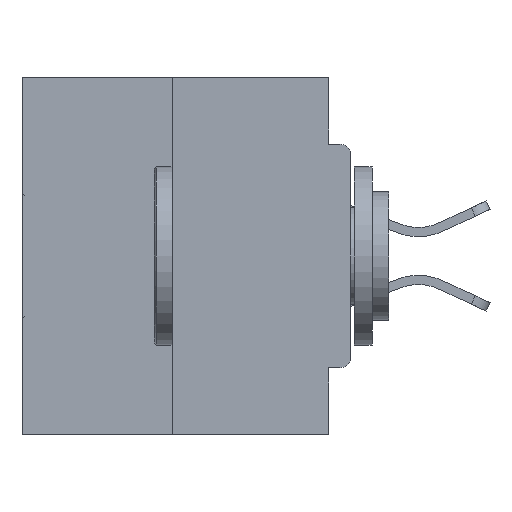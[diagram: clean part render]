
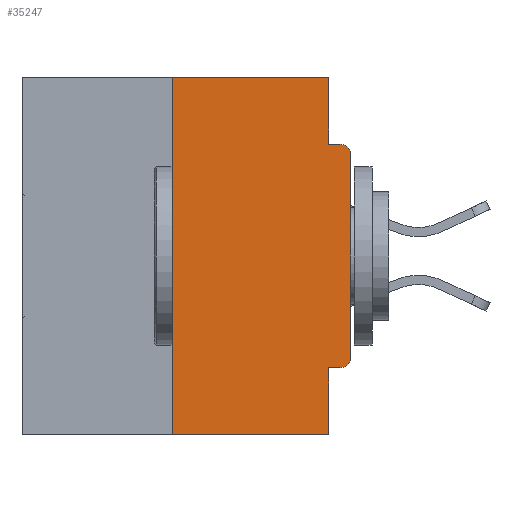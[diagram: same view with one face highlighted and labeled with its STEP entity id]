
A CAD part, left-side view. The second image highlights one B-rep face of the part: STEP entity #35247.
In plain terms, the highlighted planar face has unit normal (-1, 0, 0).
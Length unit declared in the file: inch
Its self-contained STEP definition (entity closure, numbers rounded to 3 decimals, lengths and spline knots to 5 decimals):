
#77 = EDGE_CURVE ( 'NONE', #9649, #37889, #24914, .T. ) ;
#428 = CARTESIAN_POINT ( 'NONE',  ( 0., 0.015, -0.0935 ) ) ;
#820 = VECTOR ( 'NONE', #9782, 39.37008 ) ;
#1702 = ORIENTED_EDGE ( 'NONE', *, *, #34975, .T. ) ;
#1789 = DIRECTION ( 'NONE',  ( 0., 0., -1. ) ) ;
#1977 = EDGE_LOOP ( 'NONE', ( #29689, #5391, #35841, #12767, #23916, #32589, #29078, #1702, #37087, #10829 ) ) ;
#2191 = DIRECTION ( 'NONE',  ( 1., 0., 0. ) ) ;
#2637 = EDGE_CURVE ( 'NONE', #10402, #9649, #33397, .T. ) ;
#3209 = CARTESIAN_POINT ( 'NONE',  ( 0., 0.25, -0.5 ) ) ;
#3486 = DIRECTION ( 'NONE',  ( 0., 0., -1. ) ) ;
#3772 = CIRCLE ( 'NONE', #35389, 0.015 ) ;
#4325 = CARTESIAN_POINT ( 'NONE',  ( 0., 0.031, -0.5 ) ) ;
#5368 = LINE ( 'NONE', #16459, #820 ) ;
#5391 = ORIENTED_EDGE ( 'NONE', *, *, #27818, .F. ) ;
#5663 = CARTESIAN_POINT ( 'NONE',  ( 0., 0.031, -0.5 ) ) ;
#6041 = EDGE_CURVE ( 'NONE', #34125, #19126, #41507, .T. ) ;
#6075 = VERTEX_POINT ( 'NONE', #8174 ) ;
#6329 = LINE ( 'NONE', #6885, #13990 ) ;
#6885 = CARTESIAN_POINT ( 'NONE',  ( 0., 0.25, 0. ) ) ;
#6914 = DIRECTION ( 'NONE',  ( -1., 0., 0. ) ) ;
#7132 = DIRECTION ( 'NONE',  ( 0., -1., 0. ) ) ;
#8014 = CARTESIAN_POINT ( 'NONE',  ( 0., 0.015, -0.4065 ) ) ;
#8174 = CARTESIAN_POINT ( 'NONE',  ( 0., 0.031, 0. ) ) ;
#8627 = EDGE_CURVE ( 'NONE', #26573, #36300, #5368, .T. ) ;
#9649 = VERTEX_POINT ( 'NONE', #23839 ) ;
#9782 = DIRECTION ( 'NONE',  ( 0., 0., 1. ) ) ;
#10402 = VERTEX_POINT ( 'NONE', #8014 ) ;
#10441 = DIRECTION ( 'NONE',  ( 0., 0., -1. ) ) ;
#10829 = ORIENTED_EDGE ( 'NONE', *, *, #27573, .F. ) ;
#11449 = VECTOR ( 'NONE', #14709, 39.37008 ) ;
#12528 = CARTESIAN_POINT ( 'NONE',  ( 0., 0., -0.4065 ) ) ;
#12767 = ORIENTED_EDGE ( 'NONE', *, *, #77, .F. ) ;
#13337 = EDGE_CURVE ( 'NONE', #36938, #6075, #29462, .T. ) ;
#13501 = LINE ( 'NONE', #40836, #11449 ) ;
#13732 = DIRECTION ( 'NONE',  ( 0., 0., -1. ) ) ;
#13990 = VECTOR ( 'NONE', #35572, 39.37008 ) ;
#14709 = DIRECTION ( 'NONE',  ( 0., 0., -1. ) ) ;
#14954 = PLANE ( 'NONE',  #40174 ) ;
#15681 = EDGE_CURVE ( 'NONE', #18547, #37889, #33764, .T. ) ;
#16213 = CARTESIAN_POINT ( 'NONE',  ( 0., 0.031, -0.0935 ) ) ;
#16239 = CARTESIAN_POINT ( 'NONE',  ( 0., 0.015, -0.3915 ) ) ;
#16368 = DIRECTION ( 'NONE',  ( 0., 1., 0. ) ) ;
#16459 = CARTESIAN_POINT ( 'NONE',  ( 0., 0., 0. ) ) ;
#17943 = CARTESIAN_POINT ( 'NONE',  ( 0., 0.46, -0.5 ) ) ;
#18479 = CARTESIAN_POINT ( 'NONE',  ( 0., 0.46, 0. ) ) ;
#18547 = VERTEX_POINT ( 'NONE', #3209 ) ;
#18785 = CIRCLE ( 'NONE', #39879, 0.015 ) ;
#19126 = VERTEX_POINT ( 'NONE', #428 ) ;
#22755 = VECTOR ( 'NONE', #16368, 39.37008 ) ;
#22892 = DIRECTION ( 'NONE',  ( -1., 0., 0. ) ) ;
#23839 = CARTESIAN_POINT ( 'NONE',  ( 0., 0.031, -0.4065 ) ) ;
#23916 = ORIENTED_EDGE ( 'NONE', *, *, #2637, .F. ) ;
#24914 = LINE ( 'NONE', #4325, #36578 ) ;
#25861 = CARTESIAN_POINT ( 'NONE',  ( 0., 0.25, 0. ) ) ;
#26373 = CARTESIAN_POINT ( 'NONE',  ( 0., 0.46, 0. ) ) ;
#26573 = VERTEX_POINT ( 'NONE', #38317 ) ;
#27352 = FACE_OUTER_BOUND ( 'NONE', #1977, .T. ) ;
#27573 = EDGE_CURVE ( 'NONE', #6075, #34125, #13501, .T. ) ;
#27818 = EDGE_CURVE ( 'NONE', #18547, #36938, #6329, .T. ) ;
#27932 = VECTOR ( 'NONE', #7132, 39.37008 ) ;
#29078 = ORIENTED_EDGE ( 'NONE', *, *, #8627, .T. ) ;
#29462 = LINE ( 'NONE', #26373, #27932 ) ;
#29689 = ORIENTED_EDGE ( 'NONE', *, *, #13337, .F. ) ;
#31924 = VECTOR ( 'NONE', #40685, 39.37008 ) ;
#32589 = ORIENTED_EDGE ( 'NONE', *, *, #40079, .T. ) ;
#33106 = CARTESIAN_POINT ( 'NONE',  ( 0., 0.015, -0.1085 ) ) ;
#33397 = LINE ( 'NONE', #12528, #22755 ) ;
#33764 = LINE ( 'NONE', #17943, #38803 ) ;
#34125 = VERTEX_POINT ( 'NONE', #16213 ) ;
#34975 = EDGE_CURVE ( 'NONE', #36300, #19126, #18785, .T. ) ;
#35247 = ADVANCED_FACE ( 'NONE', ( #27352 ), #14954, .F. ) ;
#35389 = AXIS2_PLACEMENT_3D ( 'NONE', #16239, #22892, #3486 ) ;
#35572 = DIRECTION ( 'NONE',  ( 0., 0., 1. ) ) ;
#35841 = ORIENTED_EDGE ( 'NONE', *, *, #15681, .T. ) ;
#36300 = VERTEX_POINT ( 'NONE', #41671 ) ;
#36578 = VECTOR ( 'NONE', #10441, 39.37008 ) ;
#36938 = VERTEX_POINT ( 'NONE', #25861 ) ;
#37012 = DIRECTION ( 'NONE',  ( 0., -1., 0. ) ) ;
#37087 = ORIENTED_EDGE ( 'NONE', *, *, #6041, .F. ) ;
#37151 = CARTESIAN_POINT ( 'NONE',  ( 0., 0., -0.0935 ) ) ;
#37889 = VERTEX_POINT ( 'NONE', #5663 ) ;
#38317 = CARTESIAN_POINT ( 'NONE',  ( 0., 0., -0.3915 ) ) ;
#38803 = VECTOR ( 'NONE', #37012, 39.37008 ) ;
#39879 = AXIS2_PLACEMENT_3D ( 'NONE', #33106, #6914, #13732 ) ;
#40079 = EDGE_CURVE ( 'NONE', #10402, #26573, #3772, .T. ) ;
#40174 = AXIS2_PLACEMENT_3D ( 'NONE', #18479, #2191, #1789 ) ;
#40685 = DIRECTION ( 'NONE',  ( 0., -1., 0. ) ) ;
#40836 = CARTESIAN_POINT ( 'NONE',  ( 0., 0.031, 0. ) ) ;
#41507 = LINE ( 'NONE', #37151, #31924 ) ;
#41671 = CARTESIAN_POINT ( 'NONE',  ( 0., 0., -0.1085 ) ) ;
